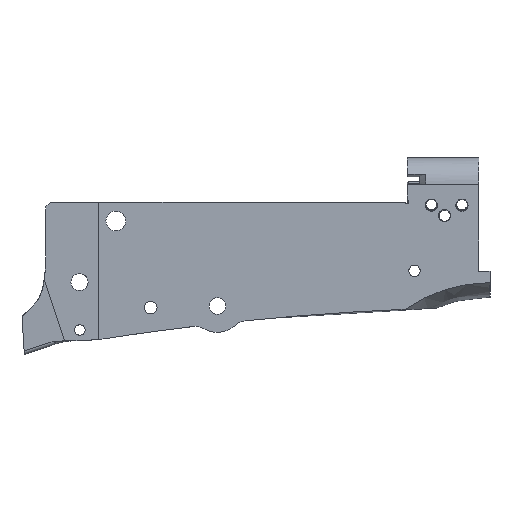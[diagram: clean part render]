
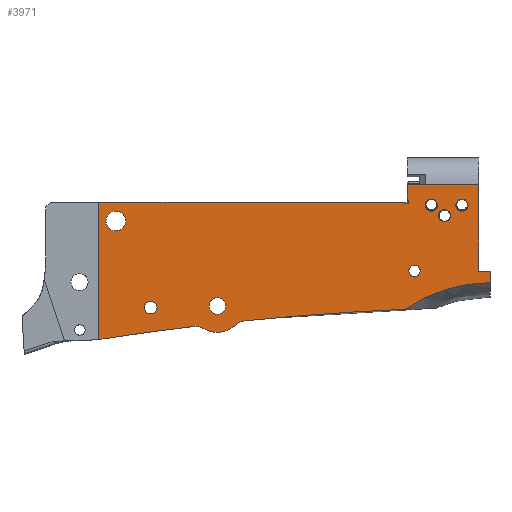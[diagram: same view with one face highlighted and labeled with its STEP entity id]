
A CAD part, left-side view. The second image highlights one B-rep face of the part: STEP entity #3971.
In plain terms, the highlighted planar face has unit normal (-1, 0, 0).
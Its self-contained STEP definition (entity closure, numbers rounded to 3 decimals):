
#147=CIRCLE('',#4084,1.85);
#149=CIRCLE('',#4086,1.85);
#152=CIRCLE('',#4090,1.85);
#155=CIRCLE('',#4093,45.79);
#156=CIRCLE('',#4097,2.5);
#217=CIRCLE('',#4229,3.);
#221=CIRCLE('',#4235,1.9);
#250=CIRCLE('',#4298,0.5);
#251=CIRCLE('',#4300,0.5);
#252=CIRCLE('',#4301,827.021);
#253=CIRCLE('',#4302,5.);
#254=CIRCLE('',#4303,8.);
#255=CIRCLE('',#4304,5.);
#256=CIRCLE('',#4305,827.021);
#257=CIRCLE('',#4306,0.5);
#258=CIRCLE('',#4307,1.75);
#309=FACE_BOUND('',#706,.T.);
#310=FACE_BOUND('',#707,.T.);
#311=FACE_BOUND('',#708,.T.);
#312=FACE_BOUND('',#709,.T.);
#313=FACE_BOUND('',#710,.T.);
#314=FACE_BOUND('',#711,.T.);
#315=FACE_BOUND('',#712,.T.);
#483=FACE_OUTER_BOUND('',#705,.T.);
#705=EDGE_LOOP('',(#3301,#3302,#3303,#3304,#3305,#3306,#3307,#3308,#3309,
#3310,#3311,#3312,#3313,#3314,#3315,#3316,#3317));
#706=EDGE_LOOP('',(#3318));
#707=EDGE_LOOP('',(#3319));
#708=EDGE_LOOP('',(#3320));
#709=EDGE_LOOP('',(#3321));
#710=EDGE_LOOP('',(#3322));
#711=EDGE_LOOP('',(#3323));
#712=EDGE_LOOP('',(#3324));
#930=LINE('',#6090,#1319);
#998=LINE('',#6417,#1387);
#1037=LINE('',#6769,#1426);
#1039=LINE('',#6776,#1428);
#1042=LINE('',#6782,#1431);
#1074=LINE('',#6907,#1463);
#1103=LINE('',#7212,#1492);
#1110=LINE('',#7238,#1499);
#1319=VECTOR('',#4693,10.);
#1387=VECTOR('',#4891,10.);
#1426=VECTOR('',#5012,10.);
#1428=VECTOR('',#5020,10.);
#1431=VECTOR('',#5027,10.);
#1463=VECTOR('',#5159,10.);
#1492=VECTOR('',#5244,10.);
#1499=VECTOR('',#5271,10.);
#1669=VERTEX_POINT('',#5823);
#1672=VERTEX_POINT('',#5898);
#1676=VERTEX_POINT('',#5958);
#1678=VERTEX_POINT('',#6019);
#1681=VERTEX_POINT('',#6041);
#1688=VERTEX_POINT('',#6060);
#1698=VERTEX_POINT('',#6087);
#1699=VERTEX_POINT('',#6089);
#1781=VERTEX_POINT('',#6406);
#1785=VERTEX_POINT('',#6415);
#1827=VERTEX_POINT('',#6767);
#1829=VERTEX_POINT('',#6775);
#1838=VERTEX_POINT('',#6808);
#1842=VERTEX_POINT('',#6820);
#1873=VERTEX_POINT('',#6905);
#1895=VERTEX_POINT('',#7209);
#1899=VERTEX_POINT('',#7221);
#1900=VERTEX_POINT('',#7222);
#1901=VERTEX_POINT('',#7227);
#1902=VERTEX_POINT('',#7229);
#1903=VERTEX_POINT('',#7231);
#1904=VERTEX_POINT('',#7233);
#1905=VERTEX_POINT('',#7235);
#1906=VERTEX_POINT('',#7240);
#2088=EDGE_CURVE('',#1669,#1669,#147,.T.);
#2092=EDGE_CURVE('',#1672,#1672,#149,.T.);
#2098=EDGE_CURVE('',#1676,#1676,#152,.T.);
#2103=EDGE_CURVE('',#1678,#1681,#155,.T.);
#2111=EDGE_CURVE('',#1688,#1688,#156,.T.);
#2125=EDGE_CURVE('',#1698,#1699,#930,.T.);
#2237=EDGE_CURVE('',#1781,#1785,#998,.F.);
#2303=EDGE_CURVE('',#1698,#1827,#1037,.T.);
#2306=EDGE_CURVE('',#1699,#1829,#1039,.T.);
#2310=EDGE_CURVE('',#1681,#1829,#1042,.T.);
#2325=EDGE_CURVE('',#1838,#1838,#217,.T.);
#2331=EDGE_CURVE('',#1842,#1842,#221,.T.);
#2373=EDGE_CURVE('',#1873,#1827,#1074,.T.);
#2415=EDGE_CURVE('',#1785,#1895,#1103,.T.);
#2420=EDGE_CURVE('',#1899,#1900,#250,.T.);
#2423=EDGE_CURVE('',#1781,#1901,#251,.T.);
#2424=EDGE_CURVE('',#1895,#1902,#252,.T.);
#2425=EDGE_CURVE('',#1903,#1902,#253,.T.);
#2426=EDGE_CURVE('',#1903,#1904,#254,.T.);
#2427=EDGE_CURVE('',#1905,#1904,#255,.T.);
#2428=EDGE_CURVE('',#1905,#1678,#256,.T.);
#2429=EDGE_CURVE('',#1873,#1900,#1110,.F.);
#2430=EDGE_CURVE('',#1899,#1901,#257,.T.);
#2431=EDGE_CURVE('',#1906,#1906,#258,.T.);
#3301=ORIENTED_EDGE('',*,*,#2423,.F.);
#3302=ORIENTED_EDGE('',*,*,#2237,.T.);
#3303=ORIENTED_EDGE('',*,*,#2415,.T.);
#3304=ORIENTED_EDGE('',*,*,#2424,.T.);
#3305=ORIENTED_EDGE('',*,*,#2425,.F.);
#3306=ORIENTED_EDGE('',*,*,#2426,.T.);
#3307=ORIENTED_EDGE('',*,*,#2427,.F.);
#3308=ORIENTED_EDGE('',*,*,#2428,.T.);
#3309=ORIENTED_EDGE('',*,*,#2103,.T.);
#3310=ORIENTED_EDGE('',*,*,#2310,.T.);
#3311=ORIENTED_EDGE('',*,*,#2306,.F.);
#3312=ORIENTED_EDGE('',*,*,#2125,.F.);
#3313=ORIENTED_EDGE('',*,*,#2303,.T.);
#3314=ORIENTED_EDGE('',*,*,#2373,.F.);
#3315=ORIENTED_EDGE('',*,*,#2429,.T.);
#3316=ORIENTED_EDGE('',*,*,#2420,.F.);
#3317=ORIENTED_EDGE('',*,*,#2430,.T.);
#3318=ORIENTED_EDGE('',*,*,#2431,.T.);
#3319=ORIENTED_EDGE('',*,*,#2331,.T.);
#3320=ORIENTED_EDGE('',*,*,#2325,.T.);
#3321=ORIENTED_EDGE('',*,*,#2111,.T.);
#3322=ORIENTED_EDGE('',*,*,#2088,.T.);
#3323=ORIENTED_EDGE('',*,*,#2092,.T.);
#3324=ORIENTED_EDGE('',*,*,#2098,.T.);
#3793=PLANE('',#4299);
#3971=ADVANCED_FACE('',(#483,#309,#310,#311,#312,#313,#314,#315),#3793,
 .F.);
#4084=AXIS2_PLACEMENT_3D('',#5824,#4631,#4632);
#4086=AXIS2_PLACEMENT_3D('',#5899,#4635,#4636);
#4090=AXIS2_PLACEMENT_3D('',#5960,#4644,#4645);
#4093=AXIS2_PLACEMENT_3D('',#6043,#4650,#4651);
#4097=AXIS2_PLACEMENT_3D('',#6061,#4665,#4666);
#4229=AXIS2_PLACEMENT_3D('',#6810,#5058,#5059);
#4235=AXIS2_PLACEMENT_3D('',#6822,#5072,#5073);
#4298=AXIS2_PLACEMENT_3D('',#7223,#5253,#5254);
#4299=AXIS2_PLACEMENT_3D('',#7226,#5257,#5258);
#4300=AXIS2_PLACEMENT_3D('',#7228,#5259,#5260);
#4301=AXIS2_PLACEMENT_3D('',#7230,#5261,#5262);
#4302=AXIS2_PLACEMENT_3D('',#7232,#5263,#5264);
#4303=AXIS2_PLACEMENT_3D('',#7234,#5265,#5266);
#4304=AXIS2_PLACEMENT_3D('',#7236,#5267,#5268);
#4305=AXIS2_PLACEMENT_3D('',#7237,#5269,#5270);
#4306=AXIS2_PLACEMENT_3D('',#7239,#5272,#5273);
#4307=AXIS2_PLACEMENT_3D('',#7241,#5274,#5275);
#4631=DIRECTION('center_axis',(1.,0.,0.));
#4632=DIRECTION('ref_axis',(0.,1.,0.));
#4635=DIRECTION('center_axis',(1.,0.,0.));
#4636=DIRECTION('ref_axis',(0.,1.,0.));
#4644=DIRECTION('center_axis',(1.,0.,0.));
#4645=DIRECTION('ref_axis',(0.,-1.,0.));
#4650=DIRECTION('center_axis',(1.,0.,0.));
#4651=DIRECTION('ref_axis',(0.,0.008,1.));
#4665=DIRECTION('center_axis',(1.,0.,0.));
#4666=DIRECTION('ref_axis',(0.,-1.,0.));
#4693=DIRECTION('',(0.,-1.,0.));
#4891=DIRECTION('',(0.,-1.,0.));
#5012=DIRECTION('',(0.,0.,1.));
#5020=DIRECTION('',(0.,0.,-1.));
#5027=DIRECTION('',(0.,-1.,0.));
#5058=DIRECTION('center_axis',(1.,0.,0.));
#5059=DIRECTION('ref_axis',(0.,1.,0.));
#5072=DIRECTION('center_axis',(1.,0.,0.));
#5073=DIRECTION('ref_axis',(0.,1.,0.));
#5159=DIRECTION('',(0.,-1.,0.));
#5244=DIRECTION('',(0.,0.,-1.));
#5253=DIRECTION('center_axis',(1.,0.,0.));
#5254=DIRECTION('ref_axis',(0.,0.866,-0.5));
#5257=DIRECTION('center_axis',(1.,0.,0.));
#5258=DIRECTION('ref_axis',(0.,1.,0.));
#5259=DIRECTION('center_axis',(1.,0.,0.));
#5260=DIRECTION('ref_axis',(0.,-0.5,0.866));
#5261=DIRECTION('center_axis',(1.,0.,0.));
#5262=DIRECTION('ref_axis',(0.,0.184,0.983));
#5263=DIRECTION('center_axis',(-1.,0.,0.));
#5264=DIRECTION('ref_axis',(0.,-0.205,0.979));
#5265=DIRECTION('center_axis',(-1.,0.,0.));
#5266=DIRECTION('ref_axis',(0.,1.,0.));
#5267=DIRECTION('center_axis',(-1.,0.,0.));
#5268=DIRECTION('ref_axis',(0.,0.415,0.91));
#5269=DIRECTION('center_axis',(1.,0.,0.));
#5270=DIRECTION('ref_axis',(0.,0.184,0.983));
#5271=DIRECTION('',(0.,0.,1.));
#5272=DIRECTION('center_axis',(1.,0.,0.));
#5273=DIRECTION('ref_axis',(0.,1.,0.));
#5274=DIRECTION('center_axis',(1.,0.,0.));
#5275=DIRECTION('ref_axis',(0.,1.,0.));
#5823=CARTESIAN_POINT('',(-16.48,14.268,37.491));
#5824=CARTESIAN_POINT('Origin',(-16.48,16.118,37.491));
#5898=CARTESIAN_POINT('',(-16.48,4.968,37.491));
#5899=CARTESIAN_POINT('Origin',(-16.48,6.818,37.491));
#5958=CARTESIAN_POINT('',(-16.48,13.918,34.291));
#5960=CARTESIAN_POINT('Origin',(-16.48,12.068,34.291));
#6019=CARTESIAN_POINT('',(-16.48,24.08,5.914));
#6041=CARTESIAN_POINT('',(-16.48,-1.532,13.989));
#6043=CARTESIAN_POINT('Origin',(-16.48,-1.889,-31.8));
#6060=CARTESIAN_POINT('',(-16.48,83.468,6.932));
#6061=CARTESIAN_POINT('Origin',(-16.48,80.968,6.932));
#6087=CARTESIAN_POINT('',(-16.48,1.668,17.422));
#6089=CARTESIAN_POINT('',(-16.48,-1.682,17.422));
#6090=CARTESIAN_POINT('',(-16.48,1.468,17.422));
#6406=CARTESIAN_POINT('',(-16.48,24.334,38.432));
#6415=CARTESIAN_POINT('',(-16.48,116.868,38.432));
#6417=CARTESIAN_POINT('',(-16.48,104.819,38.432));
#6767=CARTESIAN_POINT('',(-16.48,1.668,43.772));
#6769=CARTESIAN_POINT('',(-16.48,1.668,32.945));
#6775=CARTESIAN_POINT('',(-16.48,-1.682,13.989));
#6776=CARTESIAN_POINT('',(-16.48,-1.682,17.922));
#6782=CARTESIAN_POINT('',(-16.48,-1.532,13.989));
#6808=CARTESIAN_POINT('',(-16.48,108.768,32.682));
#6810=CARTESIAN_POINT('Origin',(-16.48,111.768,32.682));
#6820=CARTESIAN_POINT('',(-16.48,99.268,6.432));
#6822=CARTESIAN_POINT('Origin',(-16.48,101.168,6.432));
#6905=CARTESIAN_POINT('',(-16.48,23.468,43.772));
#6907=CARTESIAN_POINT('',(-16.48,23.468,43.772));
#7209=CARTESIAN_POINT('',(-16.48,116.868,-3.271));
#7212=CARTESIAN_POINT('',(-16.48,116.868,9.407));
#7221=CARTESIAN_POINT('',(-16.48,23.218,38.865));
#7222=CARTESIAN_POINT('',(-16.48,23.468,39.298));
#7223=CARTESIAN_POINT('Origin',(-16.48,22.968,39.298));
#7226=CARTESIAN_POINT('Origin',(-16.48,70.369,22.148));
#7227=CARTESIAN_POINT('',(-16.48,23.901,38.182));
#7228=CARTESIAN_POINT('Origin',(-16.48,24.334,37.932));
#7229=CARTESIAN_POINT('',(-16.48,88.176,0.701));
#7230=CARTESIAN_POINT('Origin',(-16.48,-10.864,-820.368));
#7231=CARTESIAN_POINT('',(-16.48,85.035,0.042));
#7232=CARTESIAN_POINT('Origin',(-16.48,87.577,-4.263));
#7233=CARTESIAN_POINT('',(-16.48,75.49,1.102));
#7234=CARTESIAN_POINT('Origin',(-16.48,80.968,6.932));
#7235=CARTESIAN_POINT('',(-16.48,72.57,2.433));
#7236=CARTESIAN_POINT('Origin',(-16.48,72.066,-2.542));
#7237=CARTESIAN_POINT('Origin',(-16.48,-10.864,-820.368));
#7238=CARTESIAN_POINT('',(-16.48,23.468,30.29));
#7239=CARTESIAN_POINT('Origin',(-16.48,23.468,38.432));
#7240=CARTESIAN_POINT('',(-16.48,19.468,17.522));
#7241=CARTESIAN_POINT('Origin',(-16.48,21.218,17.522));
